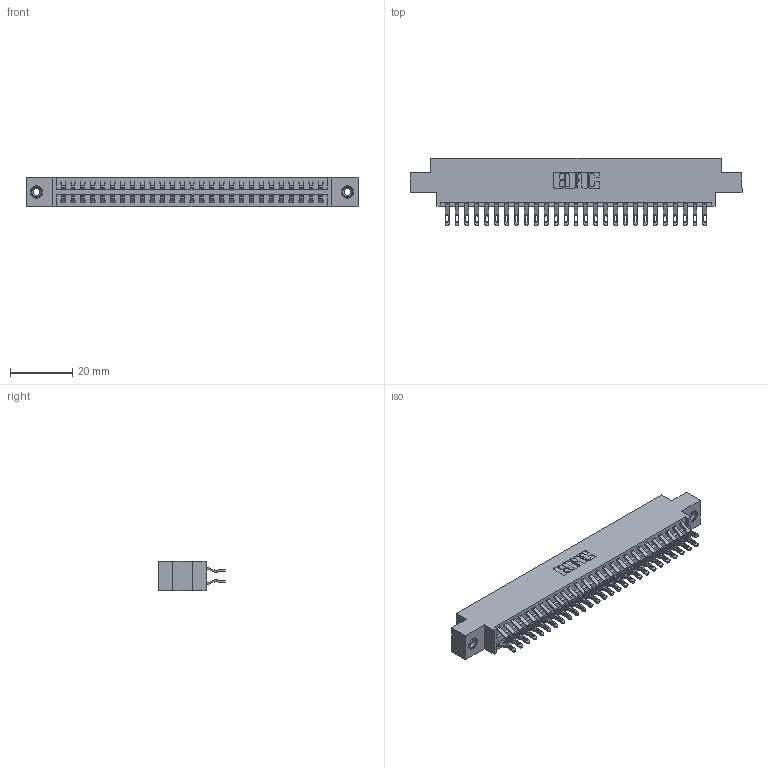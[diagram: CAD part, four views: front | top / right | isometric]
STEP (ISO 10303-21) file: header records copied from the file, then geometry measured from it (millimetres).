
FILE_DESCRIPTION (( 'STEP AP203' ), '1' );
FILE_NAME ('346-054-555-808.STEP', '2022-05-21T03:55:07', ( '' ), ( '' ), 'SwSTEP 2.0', 'SolidWorks 2020', '' );
FILE_SCHEMA (( 'CONFIG_CONTROL_DESIGN' ));
Length unit declared in the file: inch
Products named in the file (4): 346 Part_0.170 Offset - 0.156 Dia-TI; 346-054-555-808; 345-292-001_555 Tail; 345-250-001_345-250-003-102
Assembly tree (57 placements, depth 2):
  346-054-555-808
    346 Part_0.170 Offset - 0.156 Dia-TI
    345-292-001_555 Tail  x54
    345-250-001_345-250-003-102  x2
Bounding box: 106.3 x 21.46 x 9.4 mm (x, y, z)
Volume: 10244.5 mm3; surface area: 14603.9 mm2
Topology: 57 solids, 57 shells, 3318 faces, 10359 edges, 6898 vertices
Faces by surface type: plane 1894, cylinder 1408, cone 12, torus 4
Entity records: 21284 total; most frequent: CARTESIAN_POINT 3549, ORIENTED_EDGE 3446, DIRECTION 3173, EDGE_CURVE 1723, LINE 1443, VECTOR 1443, VERTEX_POINT 1144, AXIS2_PLACEMENT_3D 865
